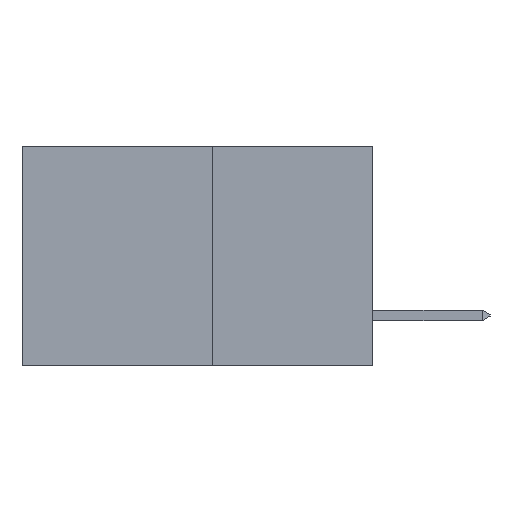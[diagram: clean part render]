
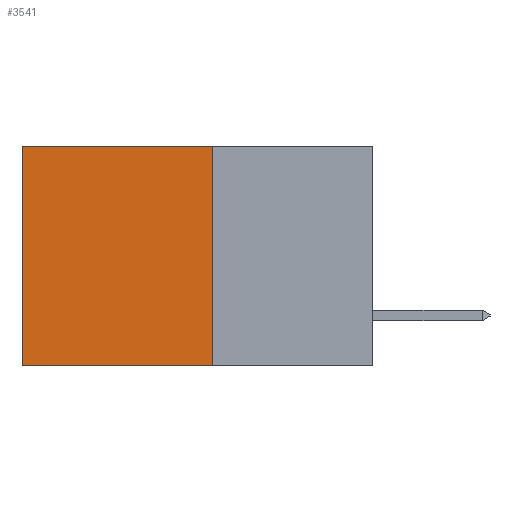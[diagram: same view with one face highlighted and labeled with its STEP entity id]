
A CAD part, left-side view. The second image highlights one B-rep face of the part: STEP entity #3541.
In plain terms, the highlighted planar face has unit normal (-1, 0, 0).
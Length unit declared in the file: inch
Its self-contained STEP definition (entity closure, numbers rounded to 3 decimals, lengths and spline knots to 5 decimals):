
#324 = VERTEX_POINT ( 'NONE', #11082 ) ;
#384 = DIRECTION ( 'NONE',  ( 0., 1., 0. ) ) ;
#486 = VECTOR ( 'NONE', #9708, 39.37008 ) ;
#1091 = CARTESIAN_POINT ( 'NONE',  ( 0.277, 0.59, -0.37 ) ) ;
#1291 = EDGE_CURVE ( 'NONE', #1913, #7298, #8264, .T. ) ;
#1292 = VERTEX_POINT ( 'NONE', #12056 ) ;
#1674 = AXIS2_PLACEMENT_3D ( 'NONE', #9470, #8849, #8309 ) ;
#1913 = VERTEX_POINT ( 'NONE', #4154 ) ;
#2113 = CARTESIAN_POINT ( 'NONE',  ( 0.277, 0.27, 0. ) ) ;
#3292 = CARTESIAN_POINT ( 'NONE',  ( 0.277, 0.59, -0.37 ) ) ;
#3541 = ADVANCED_FACE ( 'NONE', ( #9909 ), #9491, .F. ) ;
#4154 = CARTESIAN_POINT ( 'NONE',  ( 0.277, 0.27, -0.37 ) ) ;
#4451 = EDGE_CURVE ( 'NONE', #1292, #1913, #8966, .T. ) ;
#4578 = ORIENTED_EDGE ( 'NONE', *, *, #11747, .T. ) ;
#4889 = CARTESIAN_POINT ( 'NONE',  ( 0.277, 0.27, -0.37 ) ) ;
#4929 = ORIENTED_EDGE ( 'NONE', *, *, #1291, .F. ) ;
#5246 = ORIENTED_EDGE ( 'NONE', *, *, #4451, .F. ) ;
#5953 = VECTOR ( 'NONE', #384, 39.37008 ) ;
#6003 = VECTOR ( 'NONE', #8834, 39.37008 ) ;
#7173 = EDGE_LOOP ( 'NONE', ( #4578, #4929, #5246, #8476 ) ) ;
#7298 = VERTEX_POINT ( 'NONE', #1091 ) ;
#8264 = LINE ( 'NONE', #4889, #5953 ) ;
#8309 = DIRECTION ( 'NONE',  ( 0., 0., -1. ) ) ;
#8476 = ORIENTED_EDGE ( 'NONE', *, *, #10014, .T. ) ;
#8493 = LINE ( 'NONE', #2113, #486 ) ;
#8834 = DIRECTION ( 'NONE',  ( 0., 0., -1. ) ) ;
#8849 = DIRECTION ( 'NONE',  ( 1., 0., 0. ) ) ;
#8966 = LINE ( 'NONE', #11405, #10937 ) ;
#9470 = CARTESIAN_POINT ( 'NONE',  ( 0.277, 0.27, -0.37 ) ) ;
#9491 = PLANE ( 'NONE',  #1674 ) ;
#9708 = DIRECTION ( 'NONE',  ( 0., 1., 0. ) ) ;
#9909 = FACE_OUTER_BOUND ( 'NONE', #7173, .T. ) ;
#10014 = EDGE_CURVE ( 'NONE', #1292, #324, #8493, .T. ) ;
#10282 = LINE ( 'NONE', #3292, #6003 ) ;
#10937 = VECTOR ( 'NONE', #11223, 39.37008 ) ;
#11082 = CARTESIAN_POINT ( 'NONE',  ( 0.277, 0.59, 0. ) ) ;
#11223 = DIRECTION ( 'NONE',  ( 0., 0., -1. ) ) ;
#11405 = CARTESIAN_POINT ( 'NONE',  ( 0.277, 0.27, -0.37 ) ) ;
#11747 = EDGE_CURVE ( 'NONE', #324, #7298, #10282, .T. ) ;
#12056 = CARTESIAN_POINT ( 'NONE',  ( 0.277, 0.27, 0. ) ) ;
